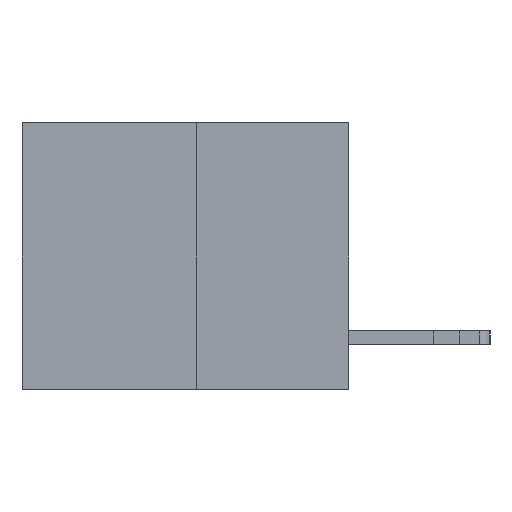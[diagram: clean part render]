
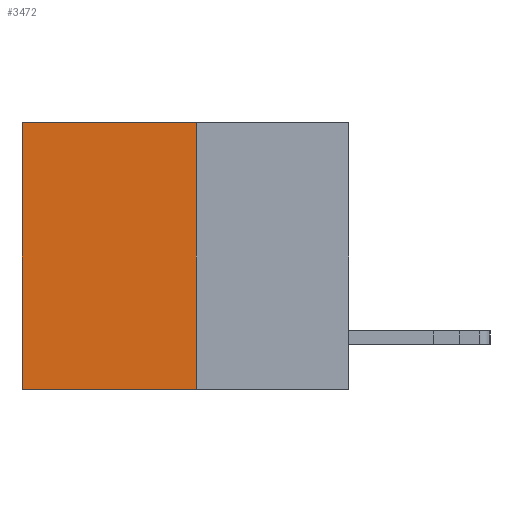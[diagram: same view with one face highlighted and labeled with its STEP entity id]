
A CAD part, left-side view. The second image highlights one B-rep face of the part: STEP entity #3472.
In plain terms, the highlighted planar face has unit normal (-1, 0, 0).
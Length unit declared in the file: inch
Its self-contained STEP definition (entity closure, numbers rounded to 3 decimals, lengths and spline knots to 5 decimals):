
#112 = CARTESIAN_POINT ( 'NONE',  ( 0.3165, 0.28, 0. ) ) ;
#294 = ORIENTED_EDGE ( 'NONE', *, *, #4887, .F. ) ;
#474 = CARTESIAN_POINT ( 'NONE',  ( 0.3165, 0.28, 0. ) ) ;
#876 = EDGE_CURVE ( 'NONE', #8196, #12058, #4147, .T. ) ;
#987 = LINE ( 'NONE', #2465, #17077 ) ;
#1398 = DIRECTION ( 'NONE',  ( 0., 0., -1. ) ) ;
#1821 = ORIENTED_EDGE ( 'NONE', *, *, #9756, .T. ) ;
#2465 = CARTESIAN_POINT ( 'NONE',  ( 0.3165, 0.28, -0.49 ) ) ;
#3472 = ADVANCED_FACE ( 'NONE', ( #16423 ), #9393, .F. ) ;
#3616 = LINE ( 'NONE', #10702, #4624 ) ;
#4147 = LINE ( 'NONE', #474, #13497 ) ;
#4624 = VECTOR ( 'NONE', #12399, 39.37008 ) ;
#4887 = EDGE_CURVE ( 'NONE', #6838, #5125, #987, .T. ) ;
#5125 = VERTEX_POINT ( 'NONE', #19258 ) ;
#6201 = CARTESIAN_POINT ( 'NONE',  ( 0.3165, 0.28, -0.49 ) ) ;
#6360 = CARTESIAN_POINT ( 'NONE',  ( 0.3165, 0.28, -0.49 ) ) ;
#6838 = VERTEX_POINT ( 'NONE', #9413 ) ;
#7738 = DIRECTION ( 'NONE',  ( 0., 0., -1. ) ) ;
#8196 = VERTEX_POINT ( 'NONE', #112 ) ;
#8732 = AXIS2_PLACEMENT_3D ( 'NONE', #6360, #14326, #1398 ) ;
#9393 = PLANE ( 'NONE',  #8732 ) ;
#9413 = CARTESIAN_POINT ( 'NONE',  ( 0.3165, 0.28, -0.49 ) ) ;
#9756 = EDGE_CURVE ( 'NONE', #12058, #5125, #3616, .T. ) ;
#9957 = EDGE_CURVE ( 'NONE', #8196, #6838, #10625, .T. ) ;
#10625 = LINE ( 'NONE', #6201, #19695 ) ;
#10702 = CARTESIAN_POINT ( 'NONE',  ( 0.3165, 0.6, -0.49 ) ) ;
#12058 = VERTEX_POINT ( 'NONE', #14173 ) ;
#12280 = ORIENTED_EDGE ( 'NONE', *, *, #876, .T. ) ;
#12399 = DIRECTION ( 'NONE',  ( 0., 0., -1. ) ) ;
#13497 = VECTOR ( 'NONE', #14741, 39.37008 ) ;
#13715 = DIRECTION ( 'NONE',  ( 0., 1., 0. ) ) ;
#14173 = CARTESIAN_POINT ( 'NONE',  ( 0.3165, 0.6, 0. ) ) ;
#14326 = DIRECTION ( 'NONE',  ( 1., 0., 0. ) ) ;
#14741 = DIRECTION ( 'NONE',  ( 0., 1., 0. ) ) ;
#15443 = EDGE_LOOP ( 'NONE', ( #1821, #294, #17236, #12280 ) ) ;
#16423 = FACE_OUTER_BOUND ( 'NONE', #15443, .T. ) ;
#17077 = VECTOR ( 'NONE', #13715, 39.37008 ) ;
#17236 = ORIENTED_EDGE ( 'NONE', *, *, #9957, .F. ) ;
#19258 = CARTESIAN_POINT ( 'NONE',  ( 0.3165, 0.6, -0.49 ) ) ;
#19695 = VECTOR ( 'NONE', #7738, 39.37008 ) ;
